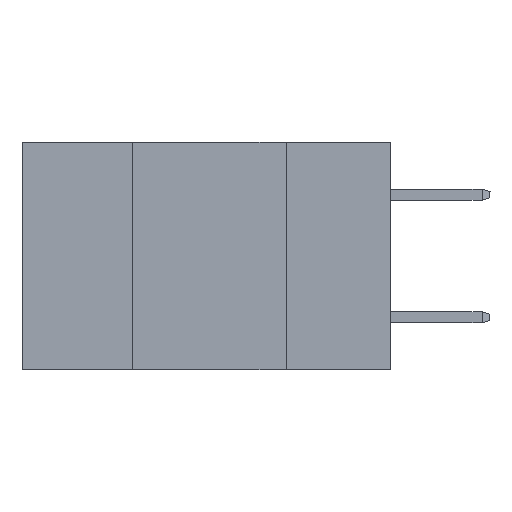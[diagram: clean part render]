
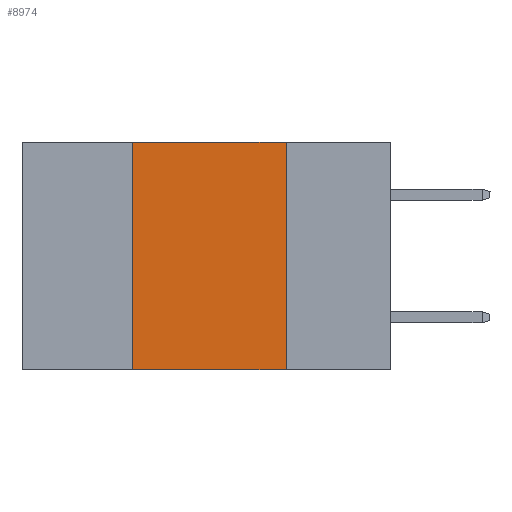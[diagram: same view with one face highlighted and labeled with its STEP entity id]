
A CAD part, left-side view. The second image highlights one B-rep face of the part: STEP entity #8974.
In plain terms, the highlighted planar face has unit normal (-1, 0, 0).
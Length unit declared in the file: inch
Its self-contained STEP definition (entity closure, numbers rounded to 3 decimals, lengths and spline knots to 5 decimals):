
#354 = ORIENTED_EDGE ( 'NONE', *, *, #14063, .F. ) ;
#867 = LINE ( 'NONE', #10686, #7685 ) ;
#1230 = VECTOR ( 'NONE', #17311, 39.37008 ) ;
#1311 = PLANE ( 'NONE',  #11712 ) ;
#1566 = CARTESIAN_POINT ( 'NONE',  ( 0., 0.6, 0. ) ) ;
#1653 = EDGE_CURVE ( 'NONE', #16218, #15966, #7139, .T. ) ;
#2194 = CARTESIAN_POINT ( 'NONE',  ( 0., 0.42, 0. ) ) ;
#3047 = VECTOR ( 'NONE', #9983, 39.37008 ) ;
#3393 = VERTEX_POINT ( 'NONE', #5525 ) ;
#3438 = ORIENTED_EDGE ( 'NONE', *, *, #23544, .F. ) ;
#4412 = EDGE_LOOP ( 'NONE', ( #21483, #354, #3438, #6323 ) ) ;
#4972 = EDGE_CURVE ( 'NONE', #3393, #15966, #18510, .T. ) ;
#5410 = CARTESIAN_POINT ( 'NONE',  ( 0., 0.17, -0.37 ) ) ;
#5525 = CARTESIAN_POINT ( 'NONE',  ( 0., 0.17, 0. ) ) ;
#6323 = ORIENTED_EDGE ( 'NONE', *, *, #1653, .T. ) ;
#7139 = LINE ( 'NONE', #11352, #1230 ) ;
#7685 = VECTOR ( 'NONE', #14623, 39.37008 ) ;
#8877 = VERTEX_POINT ( 'NONE', #13047 ) ;
#8974 = ADVANCED_FACE ( 'NONE', ( #24482 ), #1311, .F. ) ;
#9084 = DIRECTION ( 'NONE',  ( 1., 0., 0. ) ) ;
#9983 = DIRECTION ( 'NONE',  ( 0., 0., 1. ) ) ;
#10686 = CARTESIAN_POINT ( 'NONE',  ( 0., 0.6, 0. ) ) ;
#10714 = VECTOR ( 'NONE', #20526, 39.37008 ) ;
#11352 = CARTESIAN_POINT ( 'NONE',  ( 0., 0.6, -0.37 ) ) ;
#11712 = AXIS2_PLACEMENT_3D ( 'NONE', #1566, #9084, #16840 ) ;
#12789 = CARTESIAN_POINT ( 'NONE',  ( 0., 0.17, 0. ) ) ;
#13047 = CARTESIAN_POINT ( 'NONE',  ( 0., 0.42, 0. ) ) ;
#14063 = EDGE_CURVE ( 'NONE', #8877, #3393, #867, .T. ) ;
#14623 = DIRECTION ( 'NONE',  ( 0., -1., 0. ) ) ;
#15966 = VERTEX_POINT ( 'NONE', #5410 ) ;
#16218 = VERTEX_POINT ( 'NONE', #18516 ) ;
#16840 = DIRECTION ( 'NONE',  ( 0., 0., -1. ) ) ;
#17311 = DIRECTION ( 'NONE',  ( 0., -1., 0. ) ) ;
#18510 = LINE ( 'NONE', #12789, #10714 ) ;
#18516 = CARTESIAN_POINT ( 'NONE',  ( 0., 0.42, -0.37 ) ) ;
#20526 = DIRECTION ( 'NONE',  ( 0., 0., -1. ) ) ;
#21483 = ORIENTED_EDGE ( 'NONE', *, *, #4972, .F. ) ;
#21554 = LINE ( 'NONE', #2194, #3047 ) ;
#23544 = EDGE_CURVE ( 'NONE', #16218, #8877, #21554, .T. ) ;
#24482 = FACE_OUTER_BOUND ( 'NONE', #4412, .T. ) ;
